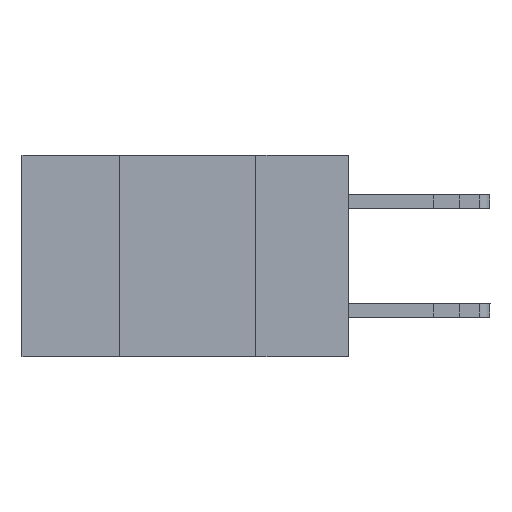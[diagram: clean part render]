
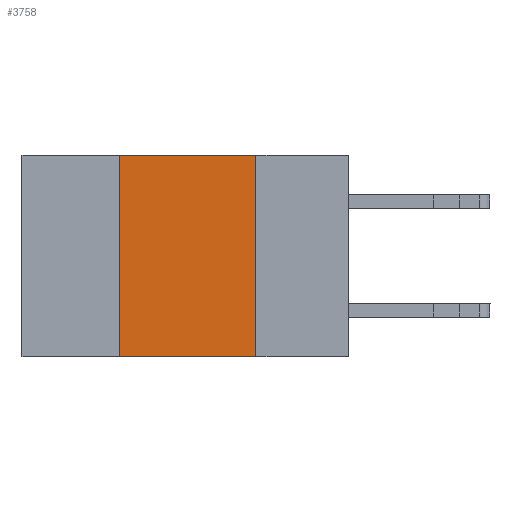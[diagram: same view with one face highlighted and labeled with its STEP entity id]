
A CAD part, left-side view. The second image highlights one B-rep face of the part: STEP entity #3758.
In plain terms, the highlighted planar face has unit normal (-1, 0, 0).
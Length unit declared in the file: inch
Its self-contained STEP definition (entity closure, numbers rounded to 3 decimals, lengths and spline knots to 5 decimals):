
#214 = EDGE_CURVE ( 'NONE', #4584, #3761, #2771, .T. ) ;
#227 = ORIENTED_EDGE ( 'NONE', *, *, #214, .F. ) ;
#1197 = DIRECTION ( 'NONE',  ( 0., 0., -1. ) ) ;
#1544 = CARTESIAN_POINT ( 'NONE',  ( 0., 0.42, -0.37 ) ) ;
#1732 = CARTESIAN_POINT ( 'NONE',  ( 0., 0.17, -0.37 ) ) ;
#2021 = CARTESIAN_POINT ( 'NONE',  ( 0., 0.17, 0. ) ) ;
#2106 = CARTESIAN_POINT ( 'NONE',  ( 0., 0.17, -0.37 ) ) ;
#2144 = ORIENTED_EDGE ( 'NONE', *, *, #9328, .F. ) ;
#2771 = LINE ( 'NONE', #1544, #10312 ) ;
#3190 = DIRECTION ( 'NONE',  ( 0., 0., -1. ) ) ;
#3320 = DIRECTION ( 'NONE',  ( 0., 0., 1. ) ) ;
#3758 = ADVANCED_FACE ( 'NONE', ( #8876 ), #4906, .F. ) ;
#3761 = VERTEX_POINT ( 'NONE', #9873 ) ;
#4072 = LINE ( 'NONE', #7015, #4343 ) ;
#4073 = CARTESIAN_POINT ( 'NONE',  ( 0., 0.42, -0.37 ) ) ;
#4343 = VECTOR ( 'NONE', #10501, 39.37008 ) ;
#4388 = VECTOR ( 'NONE', #7724, 39.37008 ) ;
#4584 = VERTEX_POINT ( 'NONE', #4073 ) ;
#4871 = ORIENTED_EDGE ( 'NONE', *, *, #5965, .F. ) ;
#4906 = PLANE ( 'NONE',  #5136 ) ;
#5046 = EDGE_LOOP ( 'NONE', ( #4871, #2144, #227, #6492 ) ) ;
#5136 = AXIS2_PLACEMENT_3D ( 'NONE', #6774, #7574, #3190 ) ;
#5784 = LINE ( 'NONE', #2106, #7010 ) ;
#5965 = EDGE_CURVE ( 'NONE', #7466, #9327, #5784, .T. ) ;
#6492 = ORIENTED_EDGE ( 'NONE', *, *, #10505, .T. ) ;
#6774 = CARTESIAN_POINT ( 'NONE',  ( 0., 0.6, 0. ) ) ;
#7010 = VECTOR ( 'NONE', #1197, 39.37008 ) ;
#7015 = CARTESIAN_POINT ( 'NONE',  ( 0., 0.6, 0. ) ) ;
#7466 = VERTEX_POINT ( 'NONE', #2021 ) ;
#7574 = DIRECTION ( 'NONE',  ( 1., 0., 0. ) ) ;
#7724 = DIRECTION ( 'NONE',  ( 0., -1., 0. ) ) ;
#7823 = LINE ( 'NONE', #11226, #4388 ) ;
#8876 = FACE_OUTER_BOUND ( 'NONE', #5046, .T. ) ;
#9327 = VERTEX_POINT ( 'NONE', #1732 ) ;
#9328 = EDGE_CURVE ( 'NONE', #3761, #7466, #4072, .T. ) ;
#9873 = CARTESIAN_POINT ( 'NONE',  ( 0., 0.42, 0. ) ) ;
#10312 = VECTOR ( 'NONE', #3320, 39.37008 ) ;
#10501 = DIRECTION ( 'NONE',  ( 0., -1., 0. ) ) ;
#10505 = EDGE_CURVE ( 'NONE', #4584, #9327, #7823, .T. ) ;
#11226 = CARTESIAN_POINT ( 'NONE',  ( 0., 0.6, -0.37 ) ) ;
